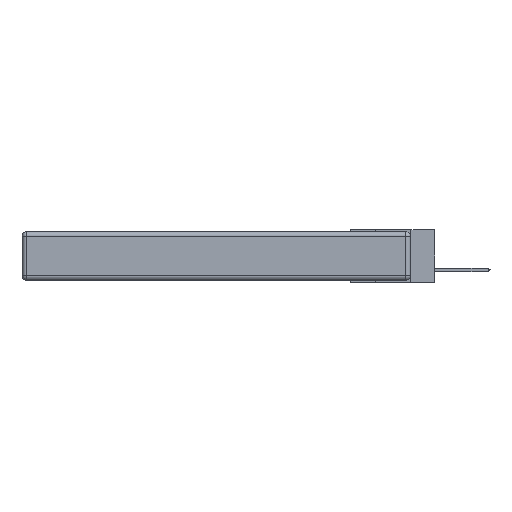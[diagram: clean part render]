
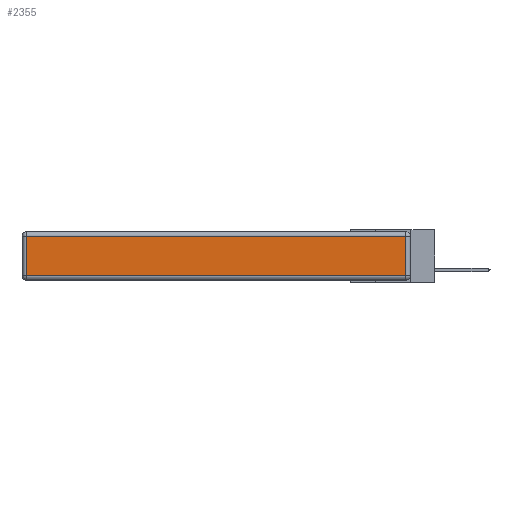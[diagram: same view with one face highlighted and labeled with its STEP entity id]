
A CAD part, left-side view. The second image highlights one B-rep face of the part: STEP entity #2355.
In plain terms, the highlighted planar face has unit normal (-1, 0, 0).
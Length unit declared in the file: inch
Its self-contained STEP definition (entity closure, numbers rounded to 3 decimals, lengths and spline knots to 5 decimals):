
#51 = EDGE_CURVE ( 'NONE', #14632, #2638, #1215, .T. ) ;
#1215 = LINE ( 'NONE', #4978, #8842 ) ;
#1307 = ORIENTED_EDGE ( 'NONE', *, *, #5208, .T. ) ;
#1419 = DIRECTION ( 'NONE',  ( 0., 0., 1. ) ) ;
#1573 = LINE ( 'NONE', #7097, #14622 ) ;
#1739 = CARTESIAN_POINT ( 'NONE',  ( 0., 2.72, -0.343 ) ) ;
#2014 = PLANE ( 'NONE',  #7011 ) ;
#2355 = ADVANCED_FACE ( 'NONE', ( #9311 ), #2014, .T. ) ;
#2638 = VERTEX_POINT ( 'NONE', #10072 ) ;
#3996 = EDGE_CURVE ( 'NONE', #2638, #9649, #7873, .T. ) ;
#4593 = ORIENTED_EDGE ( 'NONE', *, *, #51, .T. ) ;
#4978 = CARTESIAN_POINT ( 'NONE',  ( 0., 2.75, -0.03 ) ) ;
#5208 = EDGE_CURVE ( 'NONE', #9649, #13415, #9851, .T. ) ;
#5631 = EDGE_LOOP ( 'NONE', ( #1307, #6814, #4593, #9738 ) ) ;
#6462 = VECTOR ( 'NONE', #12747, 39.37008 ) ;
#6814 = ORIENTED_EDGE ( 'NONE', *, *, #10081, .T. ) ;
#7011 = AXIS2_PLACEMENT_3D ( 'NONE', #10462, #9215, #8060 ) ;
#7097 = CARTESIAN_POINT ( 'NONE',  ( 0., 0.03, -0.343 ) ) ;
#7656 = VECTOR ( 'NONE', #12628, 39.37008 ) ;
#7666 = CARTESIAN_POINT ( 'NONE',  ( 0., 0.03, -0.03 ) ) ;
#7873 = LINE ( 'NONE', #1739, #7656 ) ;
#8060 = DIRECTION ( 'NONE',  ( 0., 0., 1. ) ) ;
#8678 = CARTESIAN_POINT ( 'NONE',  ( 0., 2.72, -0.313 ) ) ;
#8767 = CARTESIAN_POINT ( 'NONE',  ( 0., 0.03, -0.313 ) ) ;
#8842 = VECTOR ( 'NONE', #13429, 39.37008 ) ;
#9215 = DIRECTION ( 'NONE',  ( -1., 0., 0. ) ) ;
#9311 = FACE_OUTER_BOUND ( 'NONE', #5631, .T. ) ;
#9649 = VERTEX_POINT ( 'NONE', #8678 ) ;
#9738 = ORIENTED_EDGE ( 'NONE', *, *, #3996, .T. ) ;
#9851 = LINE ( 'NONE', #15175, #6462 ) ;
#10072 = CARTESIAN_POINT ( 'NONE',  ( 0., 2.72, -0.03 ) ) ;
#10081 = EDGE_CURVE ( 'NONE', #13415, #14632, #1573, .T. ) ;
#10462 = CARTESIAN_POINT ( 'NONE',  ( 0., 0., -0.343 ) ) ;
#12628 = DIRECTION ( 'NONE',  ( 0., 0., -1. ) ) ;
#12747 = DIRECTION ( 'NONE',  ( 0., -1., 0. ) ) ;
#13415 = VERTEX_POINT ( 'NONE', #8767 ) ;
#13429 = DIRECTION ( 'NONE',  ( 0., 1., 0. ) ) ;
#14622 = VECTOR ( 'NONE', #1419, 39.37008 ) ;
#14632 = VERTEX_POINT ( 'NONE', #7666 ) ;
#15175 = CARTESIAN_POINT ( 'NONE',  ( 0., 0., -0.313 ) ) ;
